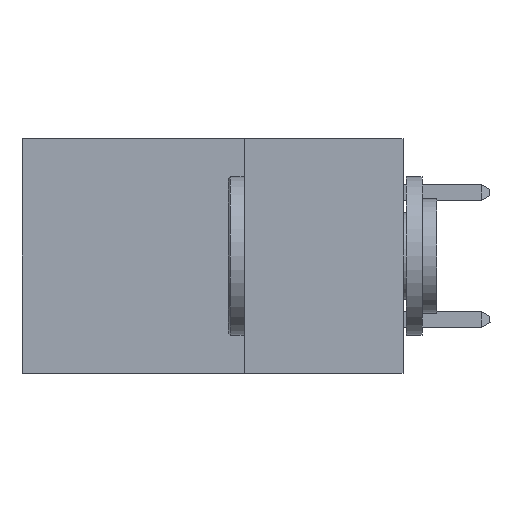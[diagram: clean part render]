
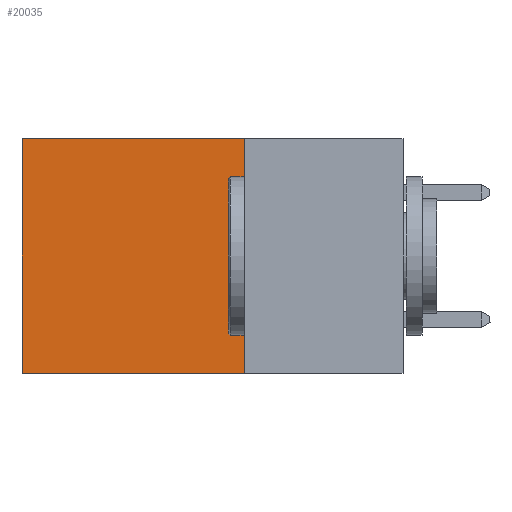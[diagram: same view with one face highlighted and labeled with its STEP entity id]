
A CAD part, left-side view. The second image highlights one B-rep face of the part: STEP entity #20035.
In plain terms, the highlighted planar face has unit normal (-1, 0, 0).
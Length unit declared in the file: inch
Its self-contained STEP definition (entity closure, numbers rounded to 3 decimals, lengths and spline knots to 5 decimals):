
#208 = FACE_OUTER_BOUND ( 'NONE', #37990, .T. ) ;
#929 = ORIENTED_EDGE ( 'NONE', *, *, #19244, .T. ) ;
#1748 = VERTEX_POINT ( 'NONE', #26245 ) ;
#3079 = EDGE_CURVE ( 'NONE', #34921, #14864, #22142, .T. ) ;
#4699 = ORIENTED_EDGE ( 'NONE', *, *, #10625, .F. ) ;
#4703 = CARTESIAN_POINT ( 'NONE',  ( 0.2875, 0.25, 0. ) ) ;
#4762 = CARTESIAN_POINT ( 'NONE',  ( 0.2875, 0.6, -0.37 ) ) ;
#4928 = VECTOR ( 'NONE', #16362, 39.37008 ) ;
#8555 = VECTOR ( 'NONE', #29648, 39.37008 ) ;
#10625 = EDGE_CURVE ( 'NONE', #30543, #34921, #34535, .T. ) ;
#11071 = CARTESIAN_POINT ( 'NONE',  ( 0.2875, 0.25, -0.37 ) ) ;
#12601 = CARTESIAN_POINT ( 'NONE',  ( 0.2875, 0.25, 0. ) ) ;
#14864 = VERTEX_POINT ( 'NONE', #4762 ) ;
#15636 = AXIS2_PLACEMENT_3D ( 'NONE', #17269, #33038, #38960 ) ;
#16362 = DIRECTION ( 'NONE',  ( 0., 0., -1. ) ) ;
#17269 = CARTESIAN_POINT ( 'NONE',  ( 0.2875, 0.25, 0. ) ) ;
#17501 = DIRECTION ( 'NONE',  ( 0., 0., -1. ) ) ;
#18005 = VECTOR ( 'NONE', #17501, 39.37008 ) ;
#19244 = EDGE_CURVE ( 'NONE', #1748, #14864, #24782, .T. ) ;
#19689 = DIRECTION ( 'NONE',  ( 0., 1., 0. ) ) ;
#20035 = ADVANCED_FACE ( 'NONE', ( #208 ), #26886, .F. ) ;
#20417 = ORIENTED_EDGE ( 'NONE', *, *, #3079, .F. ) ;
#22142 = LINE ( 'NONE', #31118, #28903 ) ;
#24782 = LINE ( 'NONE', #32129, #4928 ) ;
#26245 = CARTESIAN_POINT ( 'NONE',  ( 0.2875, 0.6, 0. ) ) ;
#26432 = CARTESIAN_POINT ( 'NONE',  ( 0.2875, 0.25, 0. ) ) ;
#26886 = PLANE ( 'NONE',  #15636 ) ;
#28903 = VECTOR ( 'NONE', #19689, 39.37008 ) ;
#29648 = DIRECTION ( 'NONE',  ( 0., 1., 0. ) ) ;
#30543 = VERTEX_POINT ( 'NONE', #12601 ) ;
#31118 = CARTESIAN_POINT ( 'NONE',  ( 0.2875, 0.25, -0.37 ) ) ;
#32129 = CARTESIAN_POINT ( 'NONE',  ( 0.2875, 0.6, 0. ) ) ;
#32628 = ORIENTED_EDGE ( 'NONE', *, *, #34961, .T. ) ;
#33038 = DIRECTION ( 'NONE',  ( 1., 0., 0. ) ) ;
#34535 = LINE ( 'NONE', #26432, #18005 ) ;
#34921 = VERTEX_POINT ( 'NONE', #11071 ) ;
#34961 = EDGE_CURVE ( 'NONE', #30543, #1748, #37673, .T. ) ;
#37673 = LINE ( 'NONE', #4703, #8555 ) ;
#37990 = EDGE_LOOP ( 'NONE', ( #929, #20417, #4699, #32628 ) ) ;
#38960 = DIRECTION ( 'NONE',  ( 0., 0., -1. ) ) ;
